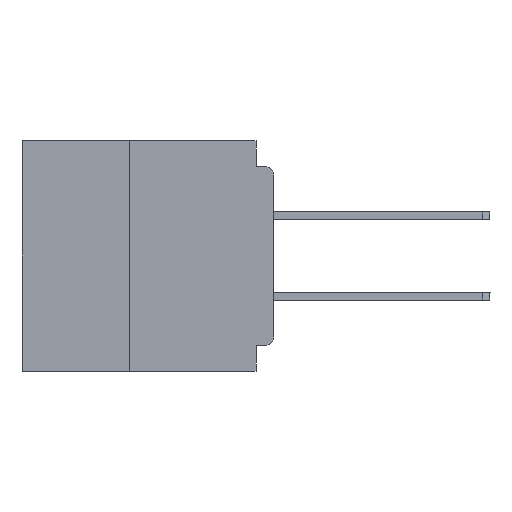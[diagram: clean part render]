
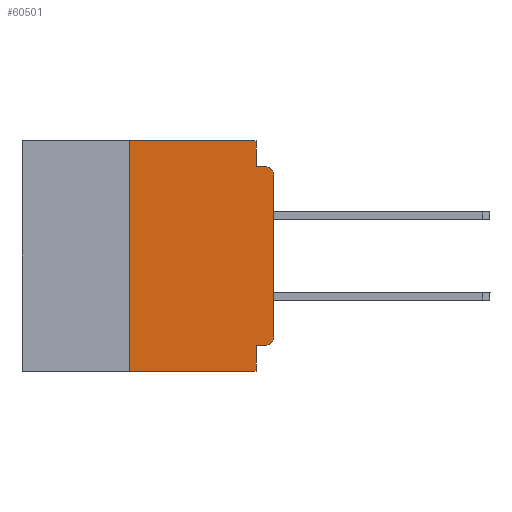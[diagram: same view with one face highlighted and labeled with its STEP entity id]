
A CAD part, left-side view. The second image highlights one B-rep face of the part: STEP entity #60501.
In plain terms, the highlighted planar face has unit normal (-1, 0, 0).
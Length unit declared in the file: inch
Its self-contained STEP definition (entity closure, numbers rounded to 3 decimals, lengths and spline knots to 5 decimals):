
#583 = VERTEX_POINT ( 'NONE', #55061 ) ;
#1181 = ORIENTED_EDGE ( 'NONE', *, *, #50959, .F. ) ;
#1736 = EDGE_CURVE ( 'NONE', #13149, #22426, #54998, .T. ) ;
#1868 = CARTESIAN_POINT ( 'NONE',  ( 0., 0.015, -0.045 ) ) ;
#4503 = DIRECTION ( 'NONE',  ( 0., -1., 0. ) ) ;
#4988 = CARTESIAN_POINT ( 'NONE',  ( 0., 0.437, 0. ) ) ;
#5072 = FACE_OUTER_BOUND ( 'NONE', #6874, .T. ) ;
#5312 = EDGE_CURVE ( 'NONE', #583, #48926, #24154, .T. ) ;
#6302 = AXIS2_PLACEMENT_3D ( 'NONE', #45981, #45928, #45846 ) ;
#6874 = EDGE_LOOP ( 'NONE', ( #7279, #39277, #56541, #45322, #62475, #1181, #57314, #25103, #43890, #50711 ) ) ;
#7279 = ORIENTED_EDGE ( 'NONE', *, *, #20926, .T. ) ;
#9988 = DIRECTION ( 'NONE',  ( 1., 0., 0. ) ) ;
#10415 = CARTESIAN_POINT ( 'NONE',  ( 0., 0.031, 0. ) ) ;
#11189 = VECTOR ( 'NONE', #43051, 39.37008 ) ;
#11504 = DIRECTION ( 'NONE',  ( -1., 0., 0. ) ) ;
#12726 = LINE ( 'NONE', #18985, #11189 ) ;
#13149 = VERTEX_POINT ( 'NONE', #60699 ) ;
#13908 = DIRECTION ( 'NONE',  ( 0., 0., -1. ) ) ;
#13911 = EDGE_CURVE ( 'NONE', #14132, #33657, #23988, .T. ) ;
#14132 = VERTEX_POINT ( 'NONE', #10415 ) ;
#16478 = VECTOR ( 'NONE', #19266, 39.37008 ) ;
#17064 = CARTESIAN_POINT ( 'NONE',  ( 0., 0.031, -0.4 ) ) ;
#18985 = CARTESIAN_POINT ( 'NONE',  ( 0., 0.437, 0. ) ) ;
#19076 = EDGE_CURVE ( 'NONE', #33657, #22426, #39197, .T. ) ;
#19266 = DIRECTION ( 'NONE',  ( 0., -1., 0. ) ) ;
#19651 = DIRECTION ( 'NONE',  ( 0., 1., 0. ) ) ;
#20898 = VECTOR ( 'NONE', #37874, 39.37008 ) ;
#20926 = EDGE_CURVE ( 'NONE', #31586, #13149, #41323, .T. ) ;
#20943 = LINE ( 'NONE', #42667, #45060 ) ;
#22426 = VERTEX_POINT ( 'NONE', #1868 ) ;
#23988 = LINE ( 'NONE', #47319, #20898 ) ;
#24154 = LINE ( 'NONE', #17064, #32440 ) ;
#25103 = ORIENTED_EDGE ( 'NONE', *, *, #5312, .F. ) ;
#25135 = CARTESIAN_POINT ( 'NONE',  ( 0., 0.25, -0.4 ) ) ;
#25970 = EDGE_CURVE ( 'NONE', #37174, #31586, #32408, .T. ) ;
#29944 = DIRECTION ( 'NONE',  ( 0., 0., 1. ) ) ;
#31575 = CARTESIAN_POINT ( 'NONE',  ( 0., 0.031, -0.045 ) ) ;
#31586 = VERTEX_POINT ( 'NONE', #32539 ) ;
#32408 = CIRCLE ( 'NONE', #54695, 0.015 ) ;
#32440 = VECTOR ( 'NONE', #13908, 39.37008 ) ;
#32539 = CARTESIAN_POINT ( 'NONE',  ( 0., 0., -0.34 ) ) ;
#32668 = LINE ( 'NONE', #48515, #58097 ) ;
#33657 = VERTEX_POINT ( 'NONE', #31575 ) ;
#33808 = AXIS2_PLACEMENT_3D ( 'NONE', #4988, #9988, #43940 ) ;
#33923 = EDGE_CURVE ( 'NONE', #61367, #14132, #12726, .T. ) ;
#34300 = PLANE ( 'NONE',  #33808 ) ;
#36136 = CARTESIAN_POINT ( 'NONE',  ( 0., 0.015, -0.355 ) ) ;
#37174 = VERTEX_POINT ( 'NONE', #36136 ) ;
#37874 = DIRECTION ( 'NONE',  ( 0., 0., -1. ) ) ;
#38504 = CARTESIAN_POINT ( 'NONE',  ( 0., 0., -0.045 ) ) ;
#39197 = LINE ( 'NONE', #38504, #16478 ) ;
#39277 = ORIENTED_EDGE ( 'NONE', *, *, #1736, .T. ) ;
#39800 = VECTOR ( 'NONE', #29944, 39.37008 ) ;
#40548 = CARTESIAN_POINT ( 'NONE',  ( 0., 0.015, -0.34 ) ) ;
#41323 = LINE ( 'NONE', #58587, #39800 ) ;
#42667 = CARTESIAN_POINT ( 'NONE',  ( 0., 0.25, -0.4 ) ) ;
#43051 = DIRECTION ( 'NONE',  ( 0., -1., 0. ) ) ;
#43449 = CARTESIAN_POINT ( 'NONE',  ( 0., 0.437, -0.4 ) ) ;
#43890 = ORIENTED_EDGE ( 'NONE', *, *, #44926, .F. ) ;
#43940 = DIRECTION ( 'NONE',  ( 0., 0., -1. ) ) ;
#44603 = VECTOR ( 'NONE', #4503, 39.37008 ) ;
#44926 = EDGE_CURVE ( 'NONE', #37174, #583, #32668, .T. ) ;
#45060 = VECTOR ( 'NONE', #47516, 39.37008 ) ;
#45322 = ORIENTED_EDGE ( 'NONE', *, *, #13911, .F. ) ;
#45402 = DIRECTION ( 'NONE',  ( 0., 0., -1. ) ) ;
#45643 = VERTEX_POINT ( 'NONE', #25135 ) ;
#45846 = DIRECTION ( 'NONE',  ( 0., 0., -1. ) ) ;
#45928 = DIRECTION ( 'NONE',  ( -1., 0., 0. ) ) ;
#45981 = CARTESIAN_POINT ( 'NONE',  ( 0., 0.015, -0.06 ) ) ;
#46066 = LINE ( 'NONE', #43449, #44603 ) ;
#47319 = CARTESIAN_POINT ( 'NONE',  ( 0., 0.031, 0. ) ) ;
#47516 = DIRECTION ( 'NONE',  ( 0., 0., 1. ) ) ;
#48515 = CARTESIAN_POINT ( 'NONE',  ( 0., 0., -0.355 ) ) ;
#48926 = VERTEX_POINT ( 'NONE', #60641 ) ;
#50711 = ORIENTED_EDGE ( 'NONE', *, *, #25970, .T. ) ;
#50959 = EDGE_CURVE ( 'NONE', #45643, #61367, #20943, .T. ) ;
#54695 = AXIS2_PLACEMENT_3D ( 'NONE', #40548, #11504, #45402 ) ;
#54998 = CIRCLE ( 'NONE', #6302, 0.015 ) ;
#55061 = CARTESIAN_POINT ( 'NONE',  ( 0., 0.031, -0.355 ) ) ;
#55126 = CARTESIAN_POINT ( 'NONE',  ( 0., 0.25, 0. ) ) ;
#56541 = ORIENTED_EDGE ( 'NONE', *, *, #19076, .F. ) ;
#57314 = ORIENTED_EDGE ( 'NONE', *, *, #61066, .T. ) ;
#58097 = VECTOR ( 'NONE', #19651, 39.37008 ) ;
#58587 = CARTESIAN_POINT ( 'NONE',  ( 0., 0., 0. ) ) ;
#60501 = ADVANCED_FACE ( 'NONE', ( #5072 ), #34300, .F. ) ;
#60641 = CARTESIAN_POINT ( 'NONE',  ( 0., 0.031, -0.4 ) ) ;
#60699 = CARTESIAN_POINT ( 'NONE',  ( 0., 0., -0.06 ) ) ;
#61066 = EDGE_CURVE ( 'NONE', #45643, #48926, #46066, .T. ) ;
#61367 = VERTEX_POINT ( 'NONE', #55126 ) ;
#62475 = ORIENTED_EDGE ( 'NONE', *, *, #33923, .F. ) ;
